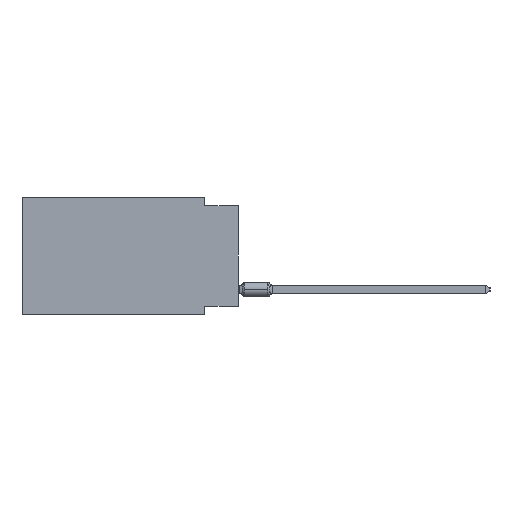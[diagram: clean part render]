
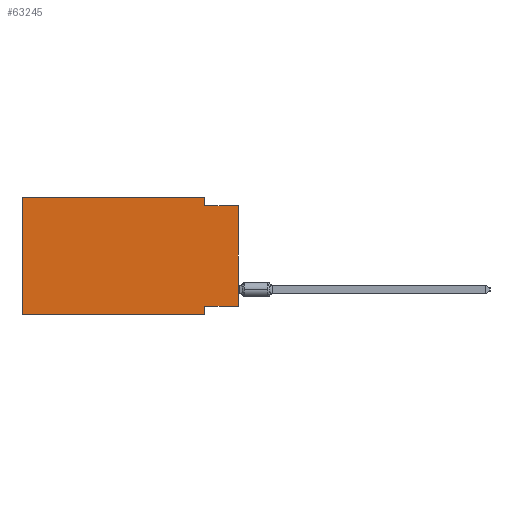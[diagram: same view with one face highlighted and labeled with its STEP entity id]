
A CAD part, left-side view. The second image highlights one B-rep face of the part: STEP entity #63245.
In plain terms, the highlighted planar face has unit normal (-1, 0, 0).
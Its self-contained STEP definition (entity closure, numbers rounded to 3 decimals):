
#540 = CARTESIAN_POINT ( 'NONE',  ( 0., 16.383, -8.89 ) ) ;
#2067 = LINE ( 'NONE', #43483, #46855 ) ;
#2233 = PLANE ( 'NONE',  #9124 ) ;
#2536 = CARTESIAN_POINT ( 'NONE',  ( 0., 0., 0. ) ) ;
#2905 = CARTESIAN_POINT ( 'NONE',  ( 0., 16.383, 0. ) ) ;
#3927 = CARTESIAN_POINT ( 'NONE',  ( 0., 16.383, -8.89 ) ) ;
#4087 = VECTOR ( 'NONE', #4912, 1000. ) ;
#4872 = LINE ( 'NONE', #9249, #18328 ) ;
#4912 = DIRECTION ( 'NONE',  ( 0., 0., 1. ) ) ;
#5241 = CARTESIAN_POINT ( 'NONE',  ( 0., 16.383, 0. ) ) ;
#6433 = ORIENTED_EDGE ( 'NONE', *, *, #10620, .T. ) ;
#8529 = LINE ( 'NONE', #18549, #46610 ) ;
#8994 = EDGE_CURVE ( 'NONE', #26715, #26803, #8529, .T. ) ;
#9124 = AXIS2_PLACEMENT_3D ( 'NONE', #2905, #52996, #28272 ) ;
#9249 = CARTESIAN_POINT ( 'NONE',  ( 0., 16.383, 0. ) ) ;
#9498 = DIRECTION ( 'NONE',  ( 0., 0., -1. ) ) ;
#10562 = VERTEX_POINT ( 'NONE', #3927 ) ;
#10620 = EDGE_CURVE ( 'NONE', #10562, #36134, #50648, .T. ) ;
#11594 = CARTESIAN_POINT ( 'NONE',  ( 0., 0., -0.635 ) ) ;
#16784 = VECTOR ( 'NONE', #42600, 1000. ) ;
#18328 = VECTOR ( 'NONE', #66014, 1000. ) ;
#18549 = CARTESIAN_POINT ( 'NONE',  ( 0., 0., -0.635 ) ) ;
#18815 = LINE ( 'NONE', #2536, #16784 ) ;
#19649 = EDGE_CURVE ( 'NONE', #53485, #26803, #18815, .T. ) ;
#19944 = DIRECTION ( 'NONE',  ( 0., -1., 0. ) ) ;
#22046 = VECTOR ( 'NONE', #19944, 1000. ) ;
#22429 = DIRECTION ( 'NONE',  ( 0., 1., 0. ) ) ;
#22952 = VERTEX_POINT ( 'NONE', #31019 ) ;
#23838 = CARTESIAN_POINT ( 'NONE',  ( 0., 2.54, -8.89 ) ) ;
#24501 = ORIENTED_EDGE ( 'NONE', *, *, #59250, .F. ) ;
#26107 = ORIENTED_EDGE ( 'NONE', *, *, #28472, .F. ) ;
#26715 = VERTEX_POINT ( 'NONE', #46003 ) ;
#26803 = VERTEX_POINT ( 'NONE', #11594 ) ;
#27680 = ORIENTED_EDGE ( 'NONE', *, *, #28223, .F. ) ;
#28183 = LINE ( 'NONE', #23838, #37176 ) ;
#28223 = EDGE_CURVE ( 'NONE', #47806, #36134, #28183, .T. ) ;
#28272 = DIRECTION ( 'NONE',  ( 0., 0., -1. ) ) ;
#28472 = EDGE_CURVE ( 'NONE', #53485, #47806, #2067, .T. ) ;
#29241 = EDGE_LOOP ( 'NONE', ( #33216, #31968, #24501, #56256, #48616, #6433, #27680, #26107 ) ) ;
#30081 = DIRECTION ( 'NONE',  ( 0., 0., -1. ) ) ;
#31019 = CARTESIAN_POINT ( 'NONE',  ( 0., 2.54, 0. ) ) ;
#31968 = ORIENTED_EDGE ( 'NONE', *, *, #8994, .F. ) ;
#33167 = CARTESIAN_POINT ( 'NONE',  ( 0., 2.54, -8.255 ) ) ;
#33216 = ORIENTED_EDGE ( 'NONE', *, *, #19649, .T. ) ;
#36134 = VERTEX_POINT ( 'NONE', #38695 ) ;
#37176 = VECTOR ( 'NONE', #30081, 1000. ) ;
#38695 = CARTESIAN_POINT ( 'NONE',  ( 0., 2.54, -8.89 ) ) ;
#39003 = EDGE_CURVE ( 'NONE', #10562, #40242, #45977, .T. ) ;
#40242 = VERTEX_POINT ( 'NONE', #47663 ) ;
#42600 = DIRECTION ( 'NONE',  ( 0., 0., 1. ) ) ;
#43427 = EDGE_CURVE ( 'NONE', #40242, #22952, #4872, .T. ) ;
#43483 = CARTESIAN_POINT ( 'NONE',  ( 0., 0., -8.255 ) ) ;
#43972 = FACE_OUTER_BOUND ( 'NONE', #29241, .T. ) ;
#45977 = LINE ( 'NONE', #5241, #4087 ) ;
#46003 = CARTESIAN_POINT ( 'NONE',  ( 0., 2.54, -0.635 ) ) ;
#46610 = VECTOR ( 'NONE', #59948, 1000. ) ;
#46855 = VECTOR ( 'NONE', #22429, 1000. ) ;
#47663 = CARTESIAN_POINT ( 'NONE',  ( 0., 16.383, 0. ) ) ;
#47806 = VERTEX_POINT ( 'NONE', #33167 ) ;
#48616 = ORIENTED_EDGE ( 'NONE', *, *, #39003, .F. ) ;
#50648 = LINE ( 'NONE', #540, #22046 ) ;
#52996 = DIRECTION ( 'NONE',  ( 1., 0., 0. ) ) ;
#53485 = VERTEX_POINT ( 'NONE', #60704 ) ;
#55251 = LINE ( 'NONE', #64639, #55661 ) ;
#55661 = VECTOR ( 'NONE', #9498, 1000. ) ;
#56256 = ORIENTED_EDGE ( 'NONE', *, *, #43427, .F. ) ;
#59250 = EDGE_CURVE ( 'NONE', #22952, #26715, #55251, .T. ) ;
#59948 = DIRECTION ( 'NONE',  ( 0., -1., 0. ) ) ;
#60704 = CARTESIAN_POINT ( 'NONE',  ( 0., 0., -8.255 ) ) ;
#63245 = ADVANCED_FACE ( 'NONE', ( #43972 ), #2233, .F. ) ;
#64639 = CARTESIAN_POINT ( 'NONE',  ( 0., 2.54, 0. ) ) ;
#66014 = DIRECTION ( 'NONE',  ( 0., -1., 0. ) ) ;
